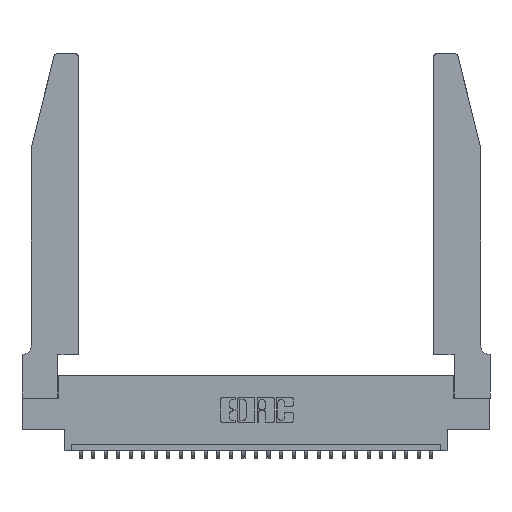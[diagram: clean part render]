
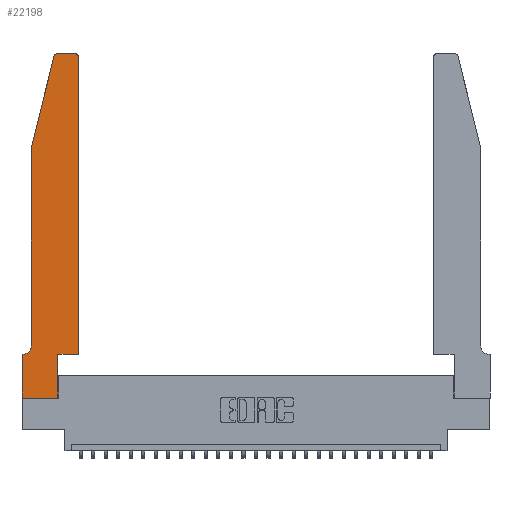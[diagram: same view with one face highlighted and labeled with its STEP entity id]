
A CAD part, top view. The second image highlights one B-rep face of the part: STEP entity #22198.
In plain terms, the highlighted planar face has unit normal (0, 0, 1).
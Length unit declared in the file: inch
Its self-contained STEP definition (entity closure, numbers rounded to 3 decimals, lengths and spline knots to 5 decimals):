
#361 = VECTOR ( 'NONE', #28110, 39.37008 ) ;
#379 = PLANE ( 'NONE',  #16746 ) ;
#409 = LINE ( 'NONE', #7983, #25265 ) ;
#516 = CARTESIAN_POINT ( 'NONE',  ( 0.0055, 0.35, 0.37 ) ) ;
#1103 = CARTESIAN_POINT ( 'NONE',  ( 0., 0., 0.37 ) ) ;
#1310 = DIRECTION ( 'NONE',  ( 0., -1., 0. ) ) ;
#1339 = VERTEX_POINT ( 'NONE', #4408 ) ;
#1677 = AXIS2_PLACEMENT_3D ( 'NONE', #13507, #15685, #2544 ) ;
#1818 = CARTESIAN_POINT ( 'NONE',  ( 0., 0.35, 0.37 ) ) ;
#1907 = ORIENTED_EDGE ( 'NONE', *, *, #7873, .T. ) ;
#2353 = CARTESIAN_POINT ( 'NONE',  ( 0.4205, 2.75, 0.37 ) ) ;
#2524 = DIRECTION ( 'NONE',  ( 0., 1., 0. ) ) ;
#2544 = DIRECTION ( 'NONE',  ( -1., 0., 0. ) ) ;
#2903 = VERTEX_POINT ( 'NONE', #2353 ) ;
#3070 = LINE ( 'NONE', #12589, #25827 ) ;
#3093 = DIRECTION ( 'NONE',  ( 1., 0., 0. ) ) ;
#3330 = EDGE_LOOP ( 'NONE', ( #13088, #14290, #15545, #14280, #6878, #16327, #20714, #27208, #8813, #4117, #1907, #23032 ) ) ;
#3606 = VERTEX_POINT ( 'NONE', #12069 ) ;
#4037 = EDGE_CURVE ( 'NONE', #10754, #1339, #15405, .T. ) ;
#4102 = VERTEX_POINT ( 'NONE', #20567 ) ;
#4107 = VECTOR ( 'NONE', #2524, 39.37008 ) ;
#4117 = ORIENTED_EDGE ( 'NONE', *, *, #12728, .T. ) ;
#4154 = EDGE_CURVE ( 'NONE', #4102, #10754, #24438, .T. ) ;
#4161 = VERTEX_POINT ( 'NONE', #14158 ) ;
#4408 = CARTESIAN_POINT ( 'NONE',  ( 0.2865, 0.35, 0.37 ) ) ;
#4771 = DIRECTION ( 'NONE',  ( 1., 0., 0. ) ) ;
#4917 = EDGE_CURVE ( 'NONE', #19052, #7292, #15009, .T. ) ;
#5370 = CARTESIAN_POINT ( 'NONE',  ( 0.0755, 2., 0.37 ) ) ;
#5941 = VECTOR ( 'NONE', #20512, 39.37008 ) ;
#6237 = LINE ( 'NONE', #5370, #361 ) ;
#6279 = CIRCLE ( 'NONE', #8494, 0.03 ) ;
#6878 = ORIENTED_EDGE ( 'NONE', *, *, #13077, .T. ) ;
#7163 = EDGE_CURVE ( 'NONE', #13006, #4161, #11483, .T. ) ;
#7292 = VERTEX_POINT ( 'NONE', #10470 ) ;
#7873 = EDGE_CURVE ( 'NONE', #3606, #28365, #409, .T. ) ;
#7983 = CARTESIAN_POINT ( 'NONE',  ( 0.4505, 0.35, 0.37 ) ) ;
#8339 = CIRCLE ( 'NONE', #1677, 0.07 ) ;
#8494 = AXIS2_PLACEMENT_3D ( 'NONE', #18745, #26931, #24630 ) ;
#8813 = ORIENTED_EDGE ( 'NONE', *, *, #4037, .T. ) ;
#9482 = FACE_OUTER_BOUND ( 'NONE', #3330, .T. ) ;
#9976 = CARTESIAN_POINT ( 'NONE',  ( 0.0755, 2., 0.37 ) ) ;
#10470 = CARTESIAN_POINT ( 'NONE',  ( 0.0755, 0.42, 0.37 ) ) ;
#10754 = VERTEX_POINT ( 'NONE', #22103 ) ;
#11214 = VERTEX_POINT ( 'NONE', #516 ) ;
#11309 = VECTOR ( 'NONE', #4771, 39.37008 ) ;
#11483 = CIRCLE ( 'NONE', #22717, 0.03 ) ;
#12069 = CARTESIAN_POINT ( 'NONE',  ( 0.4505, 0.35, 0.37 ) ) ;
#12132 = CARTESIAN_POINT ( 'NONE',  ( 0.4505, 2.72, 0.37 ) ) ;
#12278 = VECTOR ( 'NONE', #16480, 39.37008 ) ;
#12427 = DIRECTION ( 'NONE',  ( 0., 1., 0. ) ) ;
#12589 = CARTESIAN_POINT ( 'NONE',  ( 0.2605, 2.75, 0.37 ) ) ;
#12615 = VECTOR ( 'NONE', #16186, 39.37008 ) ;
#12728 = EDGE_CURVE ( 'NONE', #1339, #3606, #17648, .T. ) ;
#13006 = VERTEX_POINT ( 'NONE', #23954 ) ;
#13048 = EDGE_CURVE ( 'NONE', #28365, #2903, #6279, .T. ) ;
#13077 = EDGE_CURVE ( 'NONE', #7292, #11214, #8339, .T. ) ;
#13088 = ORIENTED_EDGE ( 'NONE', *, *, #26687, .T. ) ;
#13353 = DIRECTION ( 'NONE',  ( 0., 0., 1. ) ) ;
#13507 = CARTESIAN_POINT ( 'NONE',  ( 0.0055, 0.42, 0.37 ) ) ;
#13636 = DIRECTION ( 'NONE',  ( 1., 0., 0. ) ) ;
#14158 = CARTESIAN_POINT ( 'NONE',  ( 0.25487, 2.72718, 0.37 ) ) ;
#14274 = VERTEX_POINT ( 'NONE', #1818 ) ;
#14280 = ORIENTED_EDGE ( 'NONE', *, *, #4917, .T. ) ;
#14290 = ORIENTED_EDGE ( 'NONE', *, *, #7163, .T. ) ;
#14996 = CARTESIAN_POINT ( 'NONE',  ( 0.0755, 2., 0.37 ) ) ;
#15009 = LINE ( 'NONE', #9976, #20219 ) ;
#15377 = DIRECTION ( 'NONE',  ( 0., 0., 1. ) ) ;
#15405 = LINE ( 'NONE', #17356, #4107 ) ;
#15545 = ORIENTED_EDGE ( 'NONE', *, *, #16600, .T. ) ;
#15685 = DIRECTION ( 'NONE',  ( 0., 0., -1. ) ) ;
#15822 = CARTESIAN_POINT ( 'NONE',  ( 0.284, 2.72, 0.37 ) ) ;
#16186 = DIRECTION ( 'NONE',  ( 0., -1., 0. ) ) ;
#16327 = ORIENTED_EDGE ( 'NONE', *, *, #19310, .T. ) ;
#16480 = DIRECTION ( 'NONE',  ( -1., 0., 0. ) ) ;
#16600 = EDGE_CURVE ( 'NONE', #4161, #19052, #6237, .T. ) ;
#16746 = AXIS2_PLACEMENT_3D ( 'NONE', #18004, #15377, #3093 ) ;
#17356 = CARTESIAN_POINT ( 'NONE',  ( 0.2865, 0.35, 0.37 ) ) ;
#17648 = LINE ( 'NONE', #18291, #5941 ) ;
#18004 = CARTESIAN_POINT ( 'NONE',  ( 0., 0.35, 0.37 ) ) ;
#18139 = LINE ( 'NONE', #1103, #12615 ) ;
#18291 = CARTESIAN_POINT ( 'NONE',  ( 0.4505, 0.35, 0.37 ) ) ;
#18745 = CARTESIAN_POINT ( 'NONE',  ( 0.4205, 2.72, 0.37 ) ) ;
#19052 = VERTEX_POINT ( 'NONE', #14996 ) ;
#19308 = EDGE_CURVE ( 'NONE', #14274, #4102, #18139, .T. ) ;
#19310 = EDGE_CURVE ( 'NONE', #11214, #14274, #24049, .T. ) ;
#20219 = VECTOR ( 'NONE', #1310, 39.37008 ) ;
#20353 = CARTESIAN_POINT ( 'NONE',  ( 0.0755, 0.35, 0.37 ) ) ;
#20512 = DIRECTION ( 'NONE',  ( 1., 0., 0. ) ) ;
#20567 = CARTESIAN_POINT ( 'NONE',  ( 0., 0., 0.37 ) ) ;
#20714 = ORIENTED_EDGE ( 'NONE', *, *, #19308, .T. ) ;
#22103 = CARTESIAN_POINT ( 'NONE',  ( 0.2865, 0., 0.37 ) ) ;
#22198 = ADVANCED_FACE ( 'NONE', ( #9482 ), #379, .T. ) ;
#22717 = AXIS2_PLACEMENT_3D ( 'NONE', #15822, #13353, #13636 ) ;
#23032 = ORIENTED_EDGE ( 'NONE', *, *, #13048, .T. ) ;
#23954 = CARTESIAN_POINT ( 'NONE',  ( 0.284, 2.75, 0.37 ) ) ;
#24049 = LINE ( 'NONE', #20353, #12278 ) ;
#24438 = LINE ( 'NONE', #27228, #11309 ) ;
#24630 = DIRECTION ( 'NONE',  ( 1., 0., 0. ) ) ;
#25265 = VECTOR ( 'NONE', #12427, 39.37008 ) ;
#25827 = VECTOR ( 'NONE', #28115, 39.37008 ) ;
#26687 = EDGE_CURVE ( 'NONE', #2903, #13006, #3070, .T. ) ;
#26931 = DIRECTION ( 'NONE',  ( 0., 0., 1. ) ) ;
#27208 = ORIENTED_EDGE ( 'NONE', *, *, #4154, .T. ) ;
#27228 = CARTESIAN_POINT ( 'NONE',  ( 0., 0., 0.37 ) ) ;
#28110 = DIRECTION ( 'NONE',  ( -0.239, -0.971, 0. ) ) ;
#28115 = DIRECTION ( 'NONE',  ( -1., 0., 0. ) ) ;
#28365 = VERTEX_POINT ( 'NONE', #12132 ) ;
